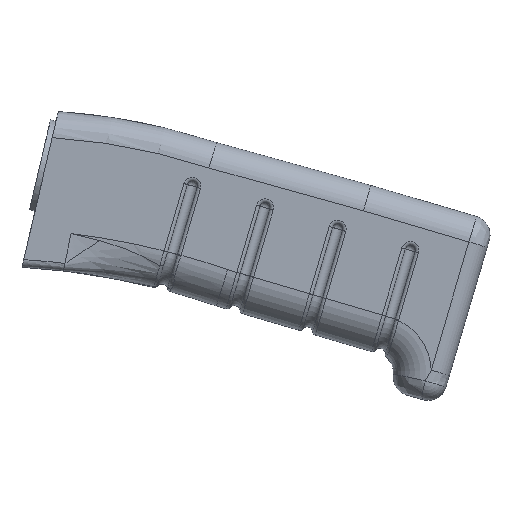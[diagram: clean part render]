
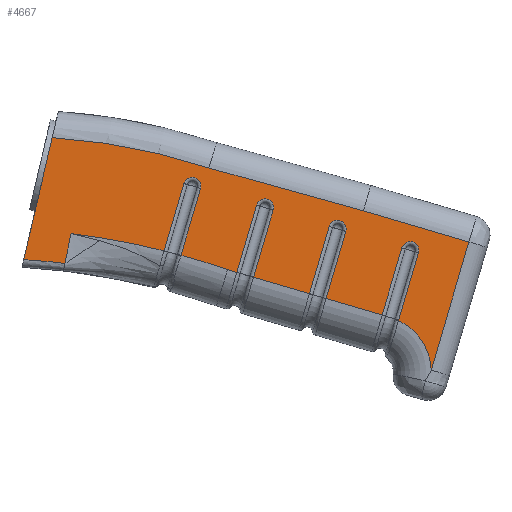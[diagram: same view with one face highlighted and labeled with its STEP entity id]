
A CAD part, top view. The second image highlights one B-rep face of the part: STEP entity #4667.
In plain terms, the highlighted planar face has unit normal (0, 0, 1).
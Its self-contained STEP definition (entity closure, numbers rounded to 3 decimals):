
#190=CIRCLE('',#4918,204.143);
#200=CIRCLE('',#4931,2.291);
#214=CIRCLE('',#4952,204.143);
#252=CIRCLE('',#5004,2.291);
#269=CIRCLE('',#5034,2.291);
#270=CIRCLE('',#5035,2.291);
#271=CIRCLE('',#5036,15.);
#272=CIRCLE('',#5037,164.532);
#273=CIRCLE('',#5038,196.143);
#490=PLANE('',#5033);
#674=FACE_OUTER_BOUND('',#962,.T.);
#962=EDGE_LOOP('',(#3942,#3943,#3944,#3945,#3946,#3947,#3948,#3949,#3950,
#3951,#3952,#3953,#3954,#3955,#3956,#3957,#3958,#3959,#3960,#3961,#3962,
#3963,#3964,#3965,#3966,#3967,#3968));
#1309=LINE('',#9336,#1612);
#1311=LINE('',#9348,#1614);
#1347=LINE('',#10066,#1650);
#1349=LINE('',#10078,#1652);
#1359=LINE('',#10126,#1662);
#1360=LINE('',#10129,#1663);
#1361=LINE('',#10131,#1664);
#1362=LINE('',#10135,#1665);
#1363=LINE('',#10137,#1666);
#1364=LINE('',#10139,#1667);
#1365=LINE('',#10143,#1668);
#1366=LINE('',#10152,#1669);
#1367=LINE('',#10154,#1670);
#1368=LINE('',#10156,#1671);
#1369=LINE('',#10160,#1672);
#1370=LINE('',#10162,#1673);
#1612=VECTOR('',#5703,10.);
#1614=VECTOR('',#5717,10.);
#1650=VECTOR('',#5887,10.);
#1652=VECTOR('',#5901,10.);
#1662=VECTOR('',#5963,10.);
#1663=VECTOR('',#5966,10.);
#1664=VECTOR('',#5967,10.);
#1665=VECTOR('',#5970,10.);
#1666=VECTOR('',#5971,10.);
#1667=VECTOR('',#5972,10.);
#1668=VECTOR('',#5975,10.);
#1669=VECTOR('',#5978,10.);
#1670=VECTOR('',#5979,10.);
#1671=VECTOR('',#5980,10.);
#1672=VECTOR('',#5983,10.);
#1673=VECTOR('',#5986,10.);
#1805=B_SPLINE_CURVE_WITH_KNOTS('',3,(#9510,#9511,#9512,#9513),
 .UNSPECIFIED.,.F.,.F.,(4,4),(0.,0.002),.UNSPECIFIED.);
#1825=B_SPLINE_CURVE_WITH_KNOTS('',3,(#10145,#10146,#10147,#10148),
 .UNSPECIFIED.,.F.,.F.,(4,4),(-0.018,0.),.UNSPECIFIED.);
#2095=VERTEX_POINT('',#9189);
#2096=VERTEX_POINT('',#9202);
#2105=VERTEX_POINT('',#9332);
#2107=VERTEX_POINT('',#9338);
#2109=VERTEX_POINT('',#9344);
#2112=VERTEX_POINT('',#9370);
#2127=VERTEX_POINT('',#9611);
#2128=VERTEX_POINT('',#9652);
#2185=VERTEX_POINT('',#10056);
#2187=VERTEX_POINT('',#10062);
#2189=VERTEX_POINT('',#10068);
#2191=VERTEX_POINT('',#10074);
#2205=VERTEX_POINT('',#10128);
#2206=VERTEX_POINT('',#10130);
#2207=VERTEX_POINT('',#10132);
#2208=VERTEX_POINT('',#10134);
#2209=VERTEX_POINT('',#10136);
#2210=VERTEX_POINT('',#10138);
#2211=VERTEX_POINT('',#10140);
#2212=VERTEX_POINT('',#10142);
#2213=VERTEX_POINT('',#10144);
#2214=VERTEX_POINT('',#10149);
#2215=VERTEX_POINT('',#10151);
#2216=VERTEX_POINT('',#10153);
#2217=VERTEX_POINT('',#10155);
#2218=VERTEX_POINT('',#10157);
#2219=VERTEX_POINT('',#10159);
#2650=EDGE_CURVE('',#2095,#2096,#190,.T.);
#2667=EDGE_CURVE('',#2096,#2105,#1309,.T.);
#2670=EDGE_CURVE('',#2105,#2107,#200,.T.);
#2673=EDGE_CURVE('',#2107,#2109,#1311,.T.);
#2688=EDGE_CURVE('',#2109,#2112,#1805,.T.);
#2702=EDGE_CURVE('',#2112,#2128,#214,.T.);
#2784=EDGE_CURVE('',#2185,#2187,#1347,.T.);
#2787=EDGE_CURVE('',#2187,#2189,#252,.T.);
#2790=EDGE_CURVE('',#2189,#2191,#1349,.T.);
#2816=EDGE_CURVE('',#2191,#2095,#1359,.T.);
#2817=EDGE_CURVE('',#2205,#2185,#1360,.T.);
#2818=EDGE_CURVE('',#2206,#2205,#1361,.T.);
#2819=EDGE_CURVE('',#2207,#2206,#269,.T.);
#2820=EDGE_CURVE('',#2208,#2207,#1362,.T.);
#2821=EDGE_CURVE('',#2209,#2208,#1363,.T.);
#2822=EDGE_CURVE('',#2210,#2209,#1364,.T.);
#2823=EDGE_CURVE('',#2211,#2210,#270,.T.);
#2824=EDGE_CURVE('',#2212,#2211,#1365,.T.);
#2825=EDGE_CURVE('',#2213,#2212,#1825,.T.);
#2826=EDGE_CURVE('',#2214,#2213,#271,.T.);
#2827=EDGE_CURVE('',#2215,#2214,#1366,.T.);
#2828=EDGE_CURVE('',#2216,#2215,#1367,.T.);
#2829=EDGE_CURVE('',#2217,#2216,#1368,.T.);
#2830=EDGE_CURVE('',#2218,#2217,#272,.T.);
#2831=EDGE_CURVE('',#2218,#2219,#1369,.T.);
#2832=EDGE_CURVE('',#2127,#2219,#273,.T.);
#2833=EDGE_CURVE('',#2127,#2128,#1370,.T.);
#3942=ORIENTED_EDGE('',*,*,#2667,.F.);
#3943=ORIENTED_EDGE('',*,*,#2650,.F.);
#3944=ORIENTED_EDGE('',*,*,#2816,.F.);
#3945=ORIENTED_EDGE('',*,*,#2790,.F.);
#3946=ORIENTED_EDGE('',*,*,#2787,.F.);
#3947=ORIENTED_EDGE('',*,*,#2784,.F.);
#3948=ORIENTED_EDGE('',*,*,#2817,.F.);
#3949=ORIENTED_EDGE('',*,*,#2818,.F.);
#3950=ORIENTED_EDGE('',*,*,#2819,.F.);
#3951=ORIENTED_EDGE('',*,*,#2820,.F.);
#3952=ORIENTED_EDGE('',*,*,#2821,.F.);
#3953=ORIENTED_EDGE('',*,*,#2822,.F.);
#3954=ORIENTED_EDGE('',*,*,#2823,.F.);
#3955=ORIENTED_EDGE('',*,*,#2824,.F.);
#3956=ORIENTED_EDGE('',*,*,#2825,.F.);
#3957=ORIENTED_EDGE('',*,*,#2826,.F.);
#3958=ORIENTED_EDGE('',*,*,#2827,.F.);
#3959=ORIENTED_EDGE('',*,*,#2828,.F.);
#3960=ORIENTED_EDGE('',*,*,#2829,.F.);
#3961=ORIENTED_EDGE('',*,*,#2830,.F.);
#3962=ORIENTED_EDGE('',*,*,#2831,.T.);
#3963=ORIENTED_EDGE('',*,*,#2832,.F.);
#3964=ORIENTED_EDGE('',*,*,#2833,.T.);
#3965=ORIENTED_EDGE('',*,*,#2702,.F.);
#3966=ORIENTED_EDGE('',*,*,#2688,.F.);
#3967=ORIENTED_EDGE('',*,*,#2673,.F.);
#3968=ORIENTED_EDGE('',*,*,#2670,.F.);
#4667=ADVANCED_FACE('',(#674),#490,.T.);
#4918=AXIS2_PLACEMENT_3D('',#9203,#5680,#5681);
#4931=AXIS2_PLACEMENT_3D('',#9342,#5710,#5711);
#4952=AXIS2_PLACEMENT_3D('',#9653,#5758,#5759);
#5004=AXIS2_PLACEMENT_3D('',#10072,#5894,#5895);
#5033=AXIS2_PLACEMENT_3D('',#10127,#5964,#5965);
#5034=AXIS2_PLACEMENT_3D('',#10133,#5968,#5969);
#5035=AXIS2_PLACEMENT_3D('',#10141,#5973,#5974);
#5036=AXIS2_PLACEMENT_3D('',#10150,#5976,#5977);
#5037=AXIS2_PLACEMENT_3D('',#10158,#5981,#5982);
#5038=AXIS2_PLACEMENT_3D('',#10161,#5984,#5985);
#5680=DIRECTION('center_axis',(0.,0.,1.));
#5681=DIRECTION('ref_axis',(0.223,0.975,0.));
#5703=DIRECTION('',(0.282,0.959,0.));
#5710=DIRECTION('center_axis',(0.,0.,1.));
#5711=DIRECTION('ref_axis',(0.282,0.959,0.));
#5717=DIRECTION('',(-0.282,-0.959,0.));
#5758=DIRECTION('center_axis',(0.,0.,1.));
#5759=DIRECTION('ref_axis',(0.223,0.975,0.));
#5887=DIRECTION('',(0.282,0.959,0.));
#5894=DIRECTION('center_axis',(0.,0.,1.));
#5895=DIRECTION('ref_axis',(0.282,0.959,0.));
#5901=DIRECTION('',(-0.282,-0.959,0.));
#5963=DIRECTION('',(-0.959,0.282,0.));
#5964=DIRECTION('center_axis',(0.,0.,1.));
#5965=DIRECTION('ref_axis',(1.,0.,0.));
#5966=DIRECTION('',(-0.959,0.282,0.));
#5967=DIRECTION('',(-0.282,-0.959,0.));
#5968=DIRECTION('center_axis',(0.,0.,1.));
#5969=DIRECTION('ref_axis',(0.282,0.959,0.));
#5970=DIRECTION('',(0.282,0.959,0.));
#5971=DIRECTION('',(-0.959,0.282,0.));
#5972=DIRECTION('',(-0.282,-0.959,0.));
#5973=DIRECTION('center_axis',(0.,0.,1.));
#5974=DIRECTION('ref_axis',(0.282,0.959,0.));
#5975=DIRECTION('',(0.282,0.959,0.));
#5976=DIRECTION('center_axis',(0.,0.,1.));
#5977=DIRECTION('ref_axis',(0.836,0.549,0.));
#5978=DIRECTION('',(-0.282,-0.959,0.));
#5979=DIRECTION('',(0.959,-0.282,0.));
#5980=DIRECTION('',(0.964,-0.267,0.));
#5981=DIRECTION('center_axis',(0.,0.,-1.));
#5982=DIRECTION('ref_axis',(0.193,0.981,0.));
#5983=DIRECTION('',(-0.227,-0.974,0.));
#5984=DIRECTION('center_axis',(0.,0.,1.));
#5985=DIRECTION('ref_axis',(0.089,0.996,0.));
#5986=DIRECTION('',(0.2,0.98,0.));
#9189=CARTESIAN_POINT('',(99.018,-77.558,33.));
#9202=CARTESIAN_POINT('',(86.663,-73.756,33.));
#9203=CARTESIAN_POINT('Origin',(32.829,-270.672,33.));
#9332=CARTESIAN_POINT('',(91.854,-56.12,33.));
#9336=CARTESIAN_POINT('',(86.63,-73.867,33.));
#9338=CARTESIAN_POINT('',(87.458,-54.826,33.));
#9342=CARTESIAN_POINT('Origin',(89.656,-55.473,33.));
#9344=CARTESIAN_POINT('',(82.234,-72.573,33.));
#9348=CARTESIAN_POINT('',(82.234,-72.573,33.));
#9370=CARTESIAN_POINT('',(82.227,-72.597,33.));
#9510=CARTESIAN_POINT('Ctrl Pts',(82.234,-72.573,33.));
#9511=CARTESIAN_POINT('Ctrl Pts',(82.232,-72.581,33.));
#9512=CARTESIAN_POINT('Ctrl Pts',(82.229,-72.589,33.));
#9513=CARTESIAN_POINT('Ctrl Pts',(82.227,-72.597,33.));
#9611=CARTESIAN_POINT('',(56.034,-75.907,33.));
#9652=CARTESIAN_POINT('',(57.641,-68.043,33.));
#9653=CARTESIAN_POINT('Origin',(32.829,-270.672,33.));
#10056=CARTESIAN_POINT('',(105.8,-79.554,33.));
#10062=CARTESIAN_POINT('',(111.023,-61.807,33.));
#10066=CARTESIAN_POINT('',(105.8,-79.554,33.));
#10068=CARTESIAN_POINT('',(106.627,-60.513,33.));
#10072=CARTESIAN_POINT('Origin',(108.825,-61.16,33.));
#10074=CARTESIAN_POINT('',(101.403,-78.26,33.));
#10078=CARTESIAN_POINT('',(101.403,-78.26,33.));
#10126=CARTESIAN_POINT('',(93.329,-75.883,33.));
#10127=CARTESIAN_POINT('Origin',(90.38,-65.685,33.));
#10128=CARTESIAN_POINT('',(120.59,-83.907,33.));
#10129=CARTESIAN_POINT('',(93.329,-75.883,33.));
#10130=CARTESIAN_POINT('',(125.813,-66.16,33.));
#10131=CARTESIAN_POINT('',(120.59,-83.907,33.));
#10132=CARTESIAN_POINT('',(130.209,-67.454,33.));
#10133=CARTESIAN_POINT('Origin',(128.011,-66.807,33.));
#10134=CARTESIAN_POINT('',(124.986,-85.201,33.));
#10135=CARTESIAN_POINT('',(124.986,-85.201,33.));
#10136=CARTESIAN_POINT('',(139.776,-89.554,33.));
#10137=CARTESIAN_POINT('',(93.329,-75.883,33.));
#10138=CARTESIAN_POINT('',(144.999,-71.807,33.));
#10139=CARTESIAN_POINT('',(139.776,-89.554,33.));
#10140=CARTESIAN_POINT('',(149.396,-73.101,33.));
#10141=CARTESIAN_POINT('Origin',(147.197,-72.454,33.));
#10142=CARTESIAN_POINT('',(144.172,-90.848,33.));
#10143=CARTESIAN_POINT('',(144.172,-90.848,33.));
#10144=CARTESIAN_POINT('',(144.123,-91.017,33.));
#10145=CARTESIAN_POINT('Ctrl Pts',(144.123,-91.017,33.));
#10146=CARTESIAN_POINT('Ctrl Pts',(144.139,-90.961,33.));
#10147=CARTESIAN_POINT('Ctrl Pts',(144.155,-90.904,33.));
#10148=CARTESIAN_POINT('Ctrl Pts',(144.172,-90.848,33.));
#10149=CARTESIAN_POINT('',(152.73,-104.09,33.));
#10150=CARTESIAN_POINT('Origin',(137.738,-104.591,33.));
#10151=CARTESIAN_POINT('',(162.695,-70.233,33.));
#10152=CARTESIAN_POINT('',(161.135,-75.536,33.));
#10153=CARTESIAN_POINT('',(134.841,-62.034,33.));
#10154=CARTESIAN_POINT('',(114.779,-56.13,33.));
#10155=CARTESIAN_POINT('',(94.05,-50.712,33.));
#10156=CARTESIAN_POINT('',(114.697,-56.443,33.));
#10157=CARTESIAN_POINT('',(52.68,-42.719,33.));
#10158=CARTESIAN_POINT('Origin',(42.412,-206.931,33.));
#10159=CARTESIAN_POINT('',(45.165,-74.918,33.));
#10160=CARTESIAN_POINT('',(54.293,-35.811,33.));
#10161=CARTESIAN_POINT('Origin',(32.829,-270.672,33.));
#10162=CARTESIAN_POINT('',(58.929,-61.737,33.));
